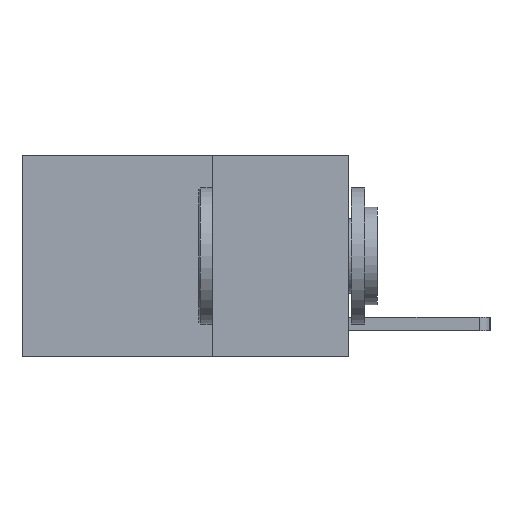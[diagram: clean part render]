
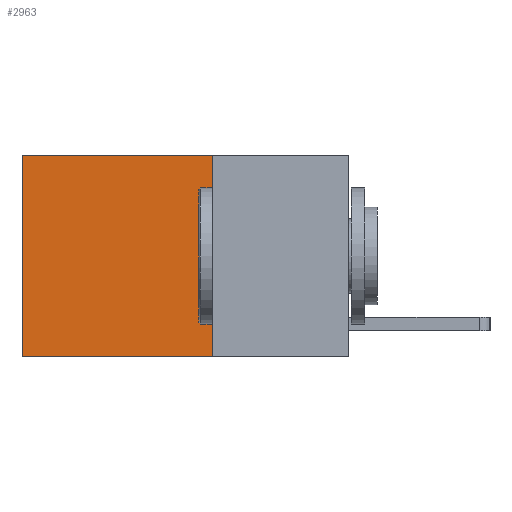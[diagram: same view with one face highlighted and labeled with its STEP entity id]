
A CAD part, left-side view. The second image highlights one B-rep face of the part: STEP entity #2963.
In plain terms, the highlighted planar face has unit normal (-1, 0, 0).
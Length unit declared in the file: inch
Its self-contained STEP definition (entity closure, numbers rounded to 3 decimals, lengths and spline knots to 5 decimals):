
#174 = CARTESIAN_POINT ( 'NONE',  ( 0.2625, 0.25, 0. ) ) ;
#254 = VERTEX_POINT ( 'NONE', #174 ) ;
#619 = DIRECTION ( 'NONE',  ( 0., 1., 0. ) ) ;
#738 = VECTOR ( 'NONE', #619, 39.37008 ) ;
#1402 = DIRECTION ( 'NONE',  ( 0., 0., -1. ) ) ;
#1735 = EDGE_CURVE ( 'NONE', #254, #2064, #4745, .T. ) ;
#1770 = EDGE_CURVE ( 'NONE', #6138, #7763, #6381, .T. ) ;
#1835 = EDGE_LOOP ( 'NONE', ( #3277, #5091, #8473, #3190 ) ) ;
#2064 = VERTEX_POINT ( 'NONE', #7273 ) ;
#2179 = EDGE_CURVE ( 'NONE', #2064, #7763, #6351, .T. ) ;
#2440 = PLANE ( 'NONE',  #6236 ) ;
#2465 = DIRECTION ( 'NONE',  ( 0., 0., -1. ) ) ;
#2754 = CARTESIAN_POINT ( 'NONE',  ( 0.2625, 0.25, 0. ) ) ;
#2852 = VECTOR ( 'NONE', #1402, 39.37008 ) ;
#2893 = VECTOR ( 'NONE', #9054, 39.37008 ) ;
#2963 = ADVANCED_FACE ( 'NONE', ( #5132 ), #2440, .F. ) ;
#3190 = ORIENTED_EDGE ( 'NONE', *, *, #1735, .T. ) ;
#3277 = ORIENTED_EDGE ( 'NONE', *, *, #2179, .T. ) ;
#4703 = LINE ( 'NONE', #7764, #2852 ) ;
#4743 = CARTESIAN_POINT ( 'NONE',  ( 0.2625, 0.6, -0.37 ) ) ;
#4745 = LINE ( 'NONE', #2754, #2893 ) ;
#5091 = ORIENTED_EDGE ( 'NONE', *, *, #1770, .F. ) ;
#5132 = FACE_OUTER_BOUND ( 'NONE', #1835, .T. ) ;
#5245 = CARTESIAN_POINT ( 'NONE',  ( 0.2625, 0.25, 0. ) ) ;
#5582 = CARTESIAN_POINT ( 'NONE',  ( 0.2625, 0.25, -0.37 ) ) ;
#6138 = VERTEX_POINT ( 'NONE', #8089 ) ;
#6236 = AXIS2_PLACEMENT_3D ( 'NONE', #5245, #6644, #2465 ) ;
#6351 = LINE ( 'NONE', #8105, #8019 ) ;
#6381 = LINE ( 'NONE', #5582, #738 ) ;
#6644 = DIRECTION ( 'NONE',  ( 1., 0., 0. ) ) ;
#7273 = CARTESIAN_POINT ( 'NONE',  ( 0.2625, 0.6, 0. ) ) ;
#7393 = DIRECTION ( 'NONE',  ( 0., 0., -1. ) ) ;
#7763 = VERTEX_POINT ( 'NONE', #4743 ) ;
#7764 = CARTESIAN_POINT ( 'NONE',  ( 0.2625, 0.25, 0. ) ) ;
#7925 = EDGE_CURVE ( 'NONE', #254, #6138, #4703, .T. ) ;
#8019 = VECTOR ( 'NONE', #7393, 39.37008 ) ;
#8089 = CARTESIAN_POINT ( 'NONE',  ( 0.2625, 0.25, -0.37 ) ) ;
#8105 = CARTESIAN_POINT ( 'NONE',  ( 0.2625, 0.6, 0. ) ) ;
#8473 = ORIENTED_EDGE ( 'NONE', *, *, #7925, .F. ) ;
#9054 = DIRECTION ( 'NONE',  ( 0., 1., 0. ) ) ;
